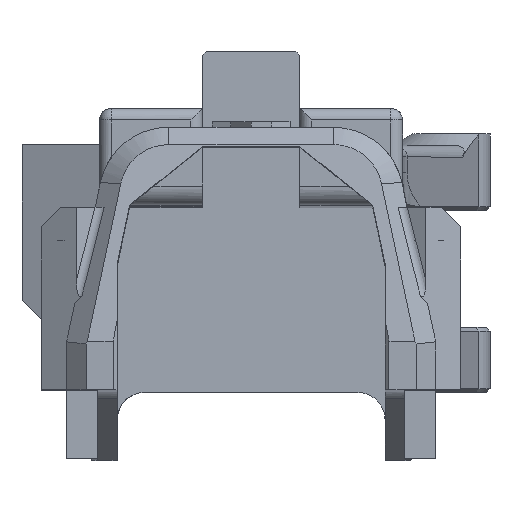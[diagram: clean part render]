
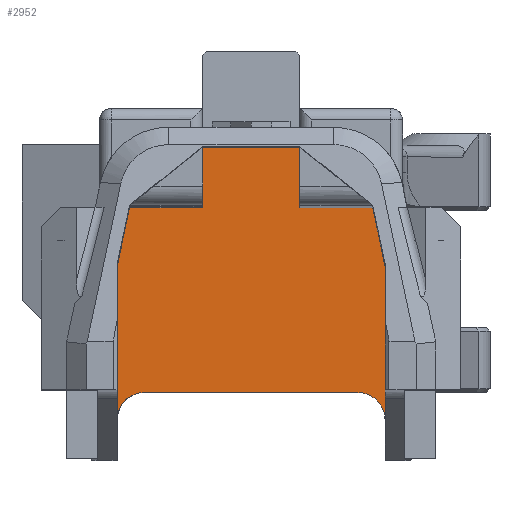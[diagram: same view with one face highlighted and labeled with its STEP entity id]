
A CAD part, top view. The second image highlights one B-rep face of the part: STEP entity #2952.
In plain terms, the highlighted planar face has unit normal (0, 0, 1).
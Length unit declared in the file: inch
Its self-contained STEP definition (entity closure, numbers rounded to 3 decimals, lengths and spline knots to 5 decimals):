
#84 = FACE_OUTER_BOUND ( 'NONE', #14317, .T. ) ;
#231 = PLANE ( 'NONE',  #1271 ) ;
#268 = LINE ( 'NONE', #12344, #14034 ) ;
#543 = VECTOR ( 'NONE', #10447, 39.37008 ) ;
#655 = LINE ( 'NONE', #9609, #11304 ) ;
#825 = CARTESIAN_POINT ( 'NONE',  ( -0.68898, 0., -8.38 ) ) ;
#1051 = VERTEX_POINT ( 'NONE', #8190 ) ;
#1090 = ORIENTED_EDGE ( 'NONE', *, *, #4775, .T. ) ;
#1187 = EDGE_CURVE ( 'NONE', #5850, #10237, #4105, .T. ) ;
#1271 = AXIS2_PLACEMENT_3D ( 'NONE', #5749, #11371, #3568 ) ;
#1451 = LINE ( 'NONE', #12227, #6849 ) ;
#1588 = LINE ( 'NONE', #12639, #8687 ) ;
#1698 = DIRECTION ( 'NONE',  ( 0., -1., 0. ) ) ;
#1780 = CARTESIAN_POINT ( 'NONE',  ( -0.68898, 0.65, -8.38 ) ) ;
#2063 = CARTESIAN_POINT ( 'NONE',  ( 0.38, 1.05, -8.38 ) ) ;
#2080 = CARTESIAN_POINT ( 'NONE',  ( -0.38, 1.05, -8.38 ) ) ;
#2461 = CARTESIAN_POINT ( 'NONE',  ( -0.25, 1.05, -8.38 ) ) ;
#2872 = CARTESIAN_POINT ( 'NONE',  ( -0.38, 1.05, -8.38 ) ) ;
#2952 = ADVANCED_FACE ( 'NONE', ( #84 ), #231, .F. ) ;
#3204 = VECTOR ( 'NONE', #10824, 39.37008 ) ;
#3225 = CARTESIAN_POINT ( 'NONE',  ( 0.38, 1.05, -8.38 ) ) ;
#3327 = EDGE_CURVE ( 'NONE', #12321, #12436, #1451, .T. ) ;
#3499 = LINE ( 'NONE', #8973, #10513 ) ;
#3563 = ORIENTED_EDGE ( 'NONE', *, *, #10554, .T. ) ;
#3568 = DIRECTION ( 'NONE',  ( -1., 0., 0. ) ) ;
#3736 = VERTEX_POINT ( 'NONE', #6074 ) ;
#3819 = EDGE_CURVE ( 'NONE', #3836, #12436, #6288, .T. ) ;
#3836 = VERTEX_POINT ( 'NONE', #2080 ) ;
#3903 = DIRECTION ( 'NONE',  ( 0., 1., 0. ) ) ;
#4016 = VECTOR ( 'NONE', #11094, 39.37008 ) ;
#4057 = EDGE_CURVE ( 'NONE', #5850, #5908, #13269, .T. ) ;
#4105 = LINE ( 'NONE', #4980, #3204 ) ;
#4629 = ORIENTED_EDGE ( 'NONE', *, *, #12224, .F. ) ;
#4771 = VERTEX_POINT ( 'NONE', #11480 ) ;
#4775 = EDGE_CURVE ( 'NONE', #6335, #13856, #1588, .T. ) ;
#4809 = CARTESIAN_POINT ( 'NONE',  ( 0.68898, -0.14, -8.38 ) ) ;
#4843 = DIRECTION ( 'NONE',  ( 0., 1., 0. ) ) ;
#4980 = CARTESIAN_POINT ( 'NONE',  ( 0.25, 0., -8.38 ) ) ;
#5095 = ORIENTED_EDGE ( 'NONE', *, *, #3327, .F. ) ;
#5121 = LINE ( 'NONE', #2872, #6333 ) ;
#5173 = CARTESIAN_POINT ( 'NONE',  ( -0.54898, -0.14, -8.38 ) ) ;
#5188 = VECTOR ( 'NONE', #9716, 39.37008 ) ;
#5235 = VERTEX_POINT ( 'NONE', #10807 ) ;
#5252 = CARTESIAN_POINT ( 'NONE',  ( -0.62521, 0.95, -8.38 ) ) ;
#5386 = ORIENTED_EDGE ( 'NONE', *, *, #4057, .T. ) ;
#5613 = DIRECTION ( 'NONE',  ( 1., 0., 0. ) ) ;
#5749 = CARTESIAN_POINT ( 'NONE',  ( 0.69882, -1.4, -8.38 ) ) ;
#5800 = EDGE_CURVE ( 'NONE', #4771, #3836, #5121, .T. ) ;
#5850 = VERTEX_POINT ( 'NONE', #14101 ) ;
#5894 = VECTOR ( 'NONE', #1698, 39.37008 ) ;
#5908 = VERTEX_POINT ( 'NONE', #3225 ) ;
#6061 = EDGE_CURVE ( 'NONE', #13856, #6159, #6935, .T. ) ;
#6074 = CARTESIAN_POINT ( 'NONE',  ( -0.68898, -0.14, -8.38 ) ) ;
#6155 = EDGE_CURVE ( 'NONE', #5908, #8072, #7580, .T. ) ;
#6159 = VERTEX_POINT ( 'NONE', #12099 ) ;
#6207 = DIRECTION ( 'NONE',  ( -0.208, -0.978, 0. ) ) ;
#6265 = LINE ( 'NONE', #825, #5894 ) ;
#6288 = LINE ( 'NONE', #9802, #12140 ) ;
#6333 = VECTOR ( 'NONE', #8623, 39.37008 ) ;
#6335 = VERTEX_POINT ( 'NONE', #4809 ) ;
#6626 = ORIENTED_EDGE ( 'NONE', *, *, #3819, .T. ) ;
#6849 = VECTOR ( 'NONE', #3903, 39.37008 ) ;
#6935 = LINE ( 'NONE', #11390, #543 ) ;
#7194 = EDGE_CURVE ( 'NONE', #8072, #4771, #3499, .T. ) ;
#7221 = ORIENTED_EDGE ( 'NONE', *, *, #7194, .T. ) ;
#7580 = LINE ( 'NONE', #2063, #4016 ) ;
#7611 = CARTESIAN_POINT ( 'NONE',  ( -0.62521, 0.95, -8.38 ) ) ;
#7765 = CARTESIAN_POINT ( 'NONE',  ( -0.25, 0.95, -8.38 ) ) ;
#8020 = DIRECTION ( 'NONE',  ( -1., 0., 0. ) ) ;
#8036 = ORIENTED_EDGE ( 'NONE', *, *, #10442, .T. ) ;
#8072 = VERTEX_POINT ( 'NONE', #12254 ) ;
#8190 = CARTESIAN_POINT ( 'NONE',  ( -0.54898, 0., -8.38 ) ) ;
#8374 = CARTESIAN_POINT ( 'NONE',  ( 0.54898, -0.14, -8.38 ) ) ;
#8385 = LINE ( 'NONE', #1780, #9702 ) ;
#8412 = ORIENTED_EDGE ( 'NONE', *, *, #1187, .F. ) ;
#8500 = VERTEX_POINT ( 'NONE', #12091 ) ;
#8623 = DIRECTION ( 'NONE',  ( 0., -1., 0. ) ) ;
#8687 = VECTOR ( 'NONE', #4843, 39.37008 ) ;
#8830 = CARTESIAN_POINT ( 'NONE',  ( 0.25, 1.05, -8.38 ) ) ;
#8867 = ORIENTED_EDGE ( 'NONE', *, *, #9371, .T. ) ;
#8877 = VECTOR ( 'NONE', #5613, 39.37008 ) ;
#8973 = CARTESIAN_POINT ( 'NONE',  ( 0.38, 1.31, -8.38 ) ) ;
#9082 = ORIENTED_EDGE ( 'NONE', *, *, #11344, .T. ) ;
#9155 = DIRECTION ( 'NONE',  ( -1., 0., 0. ) ) ;
#9317 = EDGE_CURVE ( 'NONE', #6335, #5235, #12178, .T. ) ;
#9371 = EDGE_CURVE ( 'NONE', #8500, #3736, #6265, .T. ) ;
#9460 = EDGE_CURVE ( 'NONE', #1051, #3736, #12650, .T. ) ;
#9609 = CARTESIAN_POINT ( 'NONE',  ( -0.54898, 0., -8.38 ) ) ;
#9638 = DIRECTION ( 'NONE',  ( 1., 0., 0. ) ) ;
#9702 = VECTOR ( 'NONE', #6207, 39.37008 ) ;
#9716 = DIRECTION ( 'NONE',  ( -1., 0., 0. ) ) ;
#9802 = CARTESIAN_POINT ( 'NONE',  ( -0.25, 1.05, -8.38 ) ) ;
#10021 = CARTESIAN_POINT ( 'NONE',  ( 0.68898, 0.65, -8.38 ) ) ;
#10224 = VERTEX_POINT ( 'NONE', #7611 ) ;
#10237 = VERTEX_POINT ( 'NONE', #13288 ) ;
#10442 = EDGE_CURVE ( 'NONE', #12321, #10224, #268, .T. ) ;
#10447 = DIRECTION ( 'NONE',  ( -0.208, 0.978, 0. ) ) ;
#10513 = VECTOR ( 'NONE', #8020, 39.37008 ) ;
#10554 = EDGE_CURVE ( 'NONE', #6159, #10237, #11886, .T. ) ;
#10557 = DIRECTION ( 'NONE',  ( -1., 0., 0. ) ) ;
#10807 = CARTESIAN_POINT ( 'NONE',  ( 0.54898, 0., -8.38 ) ) ;
#10824 = DIRECTION ( 'NONE',  ( 0., -1., 0. ) ) ;
#11094 = DIRECTION ( 'NONE',  ( 0., 1., 0. ) ) ;
#11304 = VECTOR ( 'NONE', #10557, 39.37008 ) ;
#11344 = EDGE_CURVE ( 'NONE', #10224, #8500, #8385, .T. ) ;
#11345 = ORIENTED_EDGE ( 'NONE', *, *, #5800, .T. ) ;
#11371 = DIRECTION ( 'NONE',  ( 0., 0., -1. ) ) ;
#11390 = CARTESIAN_POINT ( 'NONE',  ( 0.62521, 0.95, -8.38 ) ) ;
#11480 = CARTESIAN_POINT ( 'NONE',  ( -0.38, 1.31, -8.38 ) ) ;
#11816 = DIRECTION ( 'NONE',  ( 0., 0., 1. ) ) ;
#11827 = ORIENTED_EDGE ( 'NONE', *, *, #6155, .T. ) ;
#11886 = LINE ( 'NONE', #5252, #5188 ) ;
#12091 = CARTESIAN_POINT ( 'NONE',  ( -0.68898, 0.65, -8.38 ) ) ;
#12099 = CARTESIAN_POINT ( 'NONE',  ( 0.62521, 0.95, -8.38 ) ) ;
#12140 = VECTOR ( 'NONE', #14019, 39.37008 ) ;
#12178 = CIRCLE ( 'NONE', #12872, 0.14 ) ;
#12224 = EDGE_CURVE ( 'NONE', #5235, #1051, #655, .T. ) ;
#12227 = CARTESIAN_POINT ( 'NONE',  ( -0.25, 0., -8.38 ) ) ;
#12254 = CARTESIAN_POINT ( 'NONE',  ( 0.38, 1.31, -8.38 ) ) ;
#12321 = VERTEX_POINT ( 'NONE', #7765 ) ;
#12344 = CARTESIAN_POINT ( 'NONE',  ( -0.62521, 0.95, -8.38 ) ) ;
#12436 = VERTEX_POINT ( 'NONE', #2461 ) ;
#12639 = CARTESIAN_POINT ( 'NONE',  ( 0.68898, 0.65, -8.38 ) ) ;
#12650 = CIRCLE ( 'NONE', #14043, 0.14 ) ;
#12872 = AXIS2_PLACEMENT_3D ( 'NONE', #8374, #13858, #9638 ) ;
#12894 = ORIENTED_EDGE ( 'NONE', *, *, #6061, .T. ) ;
#12903 = ORIENTED_EDGE ( 'NONE', *, *, #9460, .F. ) ;
#12971 = DIRECTION ( 'NONE',  ( -1., 0., 0. ) ) ;
#13269 = LINE ( 'NONE', #8830, #8877 ) ;
#13288 = CARTESIAN_POINT ( 'NONE',  ( 0.25, 0.95, -8.38 ) ) ;
#13856 = VERTEX_POINT ( 'NONE', #10021 ) ;
#13858 = DIRECTION ( 'NONE',  ( 0., 0., 1. ) ) ;
#14019 = DIRECTION ( 'NONE',  ( 1., 0., 0. ) ) ;
#14034 = VECTOR ( 'NONE', #9155, 39.37008 ) ;
#14043 = AXIS2_PLACEMENT_3D ( 'NONE', #5173, #11816, #12971 ) ;
#14101 = CARTESIAN_POINT ( 'NONE',  ( 0.25, 1.05, -8.38 ) ) ;
#14212 = ORIENTED_EDGE ( 'NONE', *, *, #9317, .F. ) ;
#14317 = EDGE_LOOP ( 'NONE', ( #8867, #12903, #4629, #14212, #1090, #12894, #3563, #8412, #5386, #11827, #7221, #11345, #6626, #5095, #8036, #9082 ) ) ;
